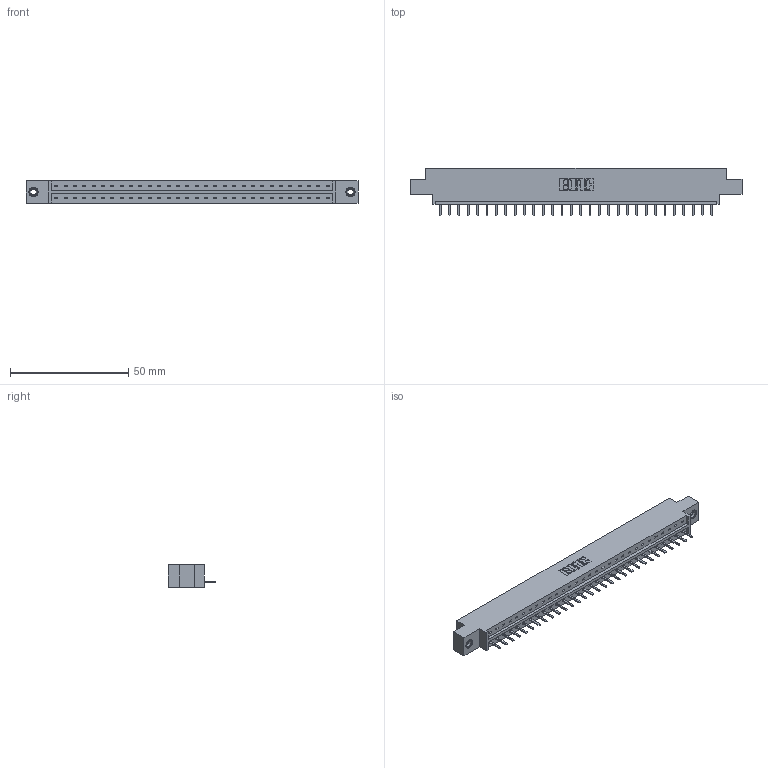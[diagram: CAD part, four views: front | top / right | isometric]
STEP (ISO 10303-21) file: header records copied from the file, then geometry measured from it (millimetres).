
FILE_DESCRIPTION (( 'STEP AP203' ), '1' );
FILE_NAME ('333-030-520-608.STEP', '2018-08-02T17:12:50', ( '' ), ( '' ), 'SwSTEP 2.0', 'SolidWorks 2016', '' );
FILE_SCHEMA (( 'CONFIG_CONTROL_DESIGN' ));
Length unit declared in the file: inch
Products named in the file (4): 345-250-001_345-250-003-102; 333-030-520-608; 333 Part_Offset - .156 Dia - TI; 345-292-001_345-293-120
Assembly tree (33 placements, depth 2):
  333-030-520-608
    333 Part_Offset - .156 Dia - TI
    345-292-001_345-293-120  x30
    345-250-001_345-250-003-102  x2
Bounding box: 140.41 x 20.02 x 9.4 mm (x, y, z)
Volume: 13705.5 mm3; surface area: 14671.7 mm2
Topology: 33 solids, 33 shells, 2038 faces, 5979 edges, 3898 vertices
Faces by surface type: plane 1426, cylinder 596, cone 12, torus 4
Entity records: 21324 total; most frequent: CARTESIAN_POINT 3675, ORIENTED_EDGE 3622, DIRECTION 3145, EDGE_CURVE 1811, VECTOR 1659, LINE 1659, VERTEX_POINT 1200, AXIS2_PLACEMENT_3D 743
